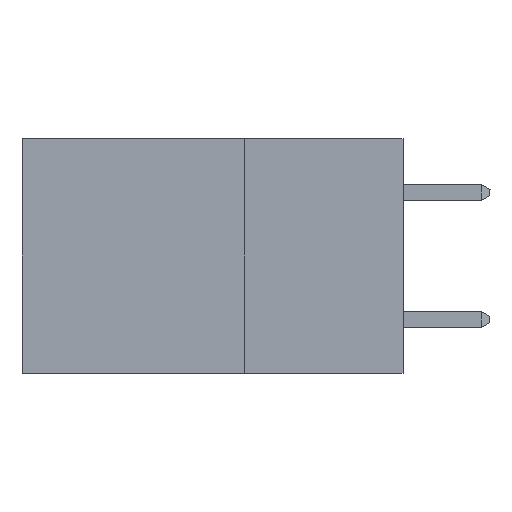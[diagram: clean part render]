
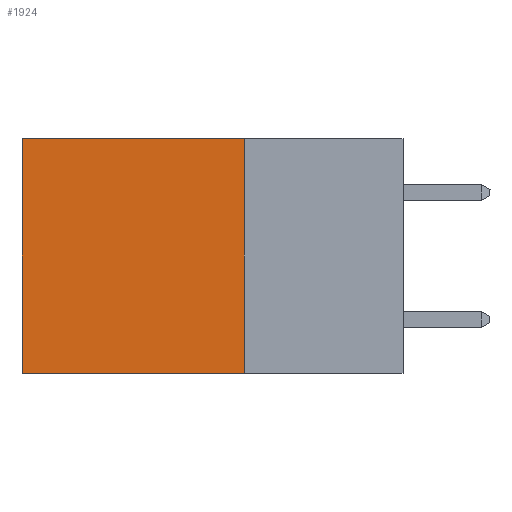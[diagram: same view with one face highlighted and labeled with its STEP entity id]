
A CAD part, left-side view. The second image highlights one B-rep face of the part: STEP entity #1924.
In plain terms, the highlighted planar face has unit normal (-1, 0, 0).
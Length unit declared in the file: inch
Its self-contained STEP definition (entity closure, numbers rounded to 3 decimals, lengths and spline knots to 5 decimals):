
#177 = ORIENTED_EDGE ( 'NONE', *, *, #13184, .F. ) ;
#1554 = AXIS2_PLACEMENT_3D ( 'NONE', #17303, #13390, #18848 ) ;
#1896 = DIRECTION ( 'NONE',  ( 0., 1., 0. ) ) ;
#1924 = ADVANCED_FACE ( 'NONE', ( #18966 ), #3894, .F. ) ;
#2470 = LINE ( 'NONE', #14238, #14661 ) ;
#3639 = VERTEX_POINT ( 'NONE', #11331 ) ;
#3894 = PLANE ( 'NONE',  #1554 ) ;
#4734 = EDGE_LOOP ( 'NONE', ( #13160, #177, #15532, #16324 ) ) ;
#5842 = EDGE_CURVE ( 'NONE', #14999, #8965, #13417, .T. ) ;
#6226 = CARTESIAN_POINT ( 'NONE',  ( 0.2875, 0.6, 0. ) ) ;
#8965 = VERTEX_POINT ( 'NONE', #13061 ) ;
#10500 = VERTEX_POINT ( 'NONE', #17744 ) ;
#11086 = VECTOR ( 'NONE', #1896, 39.37008 ) ;
#11331 = CARTESIAN_POINT ( 'NONE',  ( 0.2875, 0.6, -0.37 ) ) ;
#12230 = DIRECTION ( 'NONE',  ( 0., 1., 0. ) ) ;
#12303 = DIRECTION ( 'NONE',  ( 0., 0., -1. ) ) ;
#12332 = CARTESIAN_POINT ( 'NONE',  ( 0.2875, 0.25, 0. ) ) ;
#13061 = CARTESIAN_POINT ( 'NONE',  ( 0.2875, 0.6, 0. ) ) ;
#13160 = ORIENTED_EDGE ( 'NONE', *, *, #16976, .T. ) ;
#13184 = EDGE_CURVE ( 'NONE', #10500, #3639, #23702, .T. ) ;
#13210 = EDGE_CURVE ( 'NONE', #14999, #10500, #2470, .T. ) ;
#13390 = DIRECTION ( 'NONE',  ( 1., 0., 0. ) ) ;
#13417 = LINE ( 'NONE', #22746, #11086 ) ;
#14184 = LINE ( 'NONE', #6226, #16400 ) ;
#14238 = CARTESIAN_POINT ( 'NONE',  ( 0.2875, 0.25, 0. ) ) ;
#14661 = VECTOR ( 'NONE', #23452, 39.37008 ) ;
#14999 = VERTEX_POINT ( 'NONE', #12332 ) ;
#15532 = ORIENTED_EDGE ( 'NONE', *, *, #13210, .F. ) ;
#16324 = ORIENTED_EDGE ( 'NONE', *, *, #5842, .T. ) ;
#16400 = VECTOR ( 'NONE', #12303, 39.37008 ) ;
#16976 = EDGE_CURVE ( 'NONE', #8965, #3639, #14184, .T. ) ;
#17085 = VECTOR ( 'NONE', #12230, 39.37008 ) ;
#17303 = CARTESIAN_POINT ( 'NONE',  ( 0.2875, 0.25, 0. ) ) ;
#17744 = CARTESIAN_POINT ( 'NONE',  ( 0.2875, 0.25, -0.37 ) ) ;
#18848 = DIRECTION ( 'NONE',  ( 0., 0., -1. ) ) ;
#18966 = FACE_OUTER_BOUND ( 'NONE', #4734, .T. ) ;
#22746 = CARTESIAN_POINT ( 'NONE',  ( 0.2875, 0.25, 0. ) ) ;
#23452 = DIRECTION ( 'NONE',  ( 0., 0., -1. ) ) ;
#23702 = LINE ( 'NONE', #23955, #17085 ) ;
#23955 = CARTESIAN_POINT ( 'NONE',  ( 0.2875, 0.25, -0.37 ) ) ;
